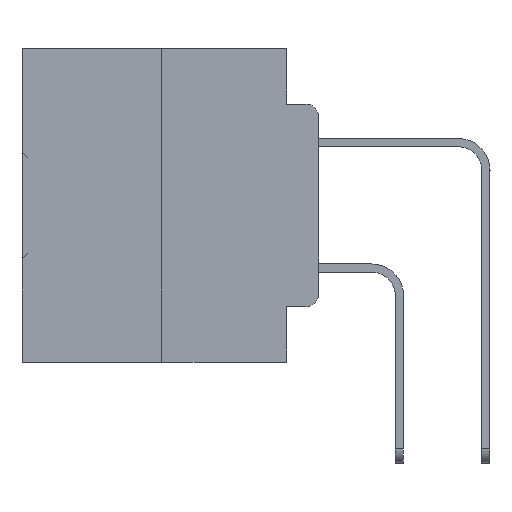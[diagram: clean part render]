
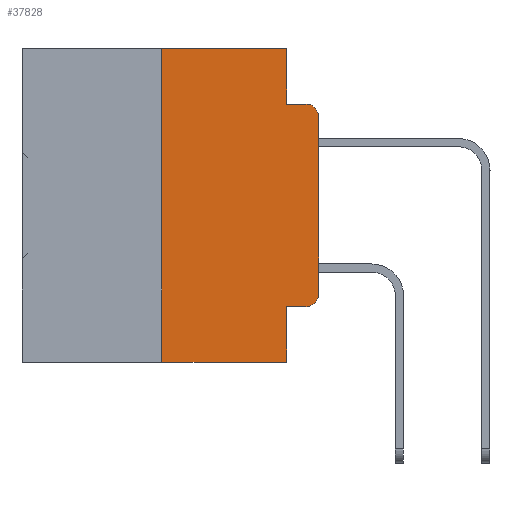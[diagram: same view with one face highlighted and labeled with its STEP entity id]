
A CAD part, left-side view. The second image highlights one B-rep face of the part: STEP entity #37828.
In plain terms, the highlighted planar face has unit normal (-1, 0, 0).
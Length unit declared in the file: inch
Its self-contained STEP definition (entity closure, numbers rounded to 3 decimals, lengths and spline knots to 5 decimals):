
#134 = DIRECTION ( 'NONE',  ( 0., 0., -1. ) ) ;
#221 = AXIS2_PLACEMENT_3D ( 'NONE', #33354, #1576, #6653 ) ;
#1245 = CARTESIAN_POINT ( 'NONE',  ( 0., 0., 0. ) ) ;
#1454 = LINE ( 'NONE', #13320, #4635 ) ;
#1519 = VERTEX_POINT ( 'NONE', #12803 ) ;
#1576 = DIRECTION ( 'NONE',  ( 1., 0., 0. ) ) ;
#2118 = CARTESIAN_POINT ( 'NONE',  ( 0., 0.473, 0. ) ) ;
#3173 = VECTOR ( 'NONE', #10102, 39.37008 ) ;
#4090 = CARTESIAN_POINT ( 'NONE',  ( 0., 0.051, 0. ) ) ;
#4349 = DIRECTION ( 'NONE',  ( 0., 0., 1. ) ) ;
#4635 = VECTOR ( 'NONE', #25233, 39.37008 ) ;
#6163 = EDGE_CURVE ( 'NONE', #16615, #1519, #25114, .T. ) ;
#6653 = DIRECTION ( 'NONE',  ( 0., 0., -1. ) ) ;
#6839 = VERTEX_POINT ( 'NONE', #30055 ) ;
#7775 = VECTOR ( 'NONE', #13465, 39.37008 ) ;
#8841 = CARTESIAN_POINT ( 'NONE',  ( 0., 0., -0.3915 ) ) ;
#9501 = DIRECTION ( 'NONE',  ( 0., 0., -1. ) ) ;
#9971 = AXIS2_PLACEMENT_3D ( 'NONE', #16643, #13518, #28905 ) ;
#10102 = DIRECTION ( 'NONE',  ( 0., 0., 1. ) ) ;
#11170 = VECTOR ( 'NONE', #9501, 39.37008 ) ;
#11258 = ORIENTED_EDGE ( 'NONE', *, *, #25419, .T. ) ;
#11680 = EDGE_CURVE ( 'NONE', #16615, #21361, #1454, .T. ) ;
#11742 = VECTOR ( 'NONE', #28440, 39.37008 ) ;
#12127 = ORIENTED_EDGE ( 'NONE', *, *, #31651, .T. ) ;
#12205 = CARTESIAN_POINT ( 'NONE',  ( 0., 0.051, 0. ) ) ;
#12661 = DIRECTION ( 'NONE',  ( 0., 0., -1. ) ) ;
#12803 = CARTESIAN_POINT ( 'NONE',  ( 0., 0.25, 0. ) ) ;
#12878 = ORIENTED_EDGE ( 'NONE', *, *, #6163, .F. ) ;
#13035 = VERTEX_POINT ( 'NONE', #8841 ) ;
#13320 = CARTESIAN_POINT ( 'NONE',  ( 0., 0.473, -0.5 ) ) ;
#13465 = DIRECTION ( 'NONE',  ( 0., -1., 0. ) ) ;
#13518 = DIRECTION ( 'NONE',  ( -1., 0., 0. ) ) ;
#15500 = CARTESIAN_POINT ( 'NONE',  ( 0., 0.051, -0.5 ) ) ;
#16203 = LINE ( 'NONE', #28486, #7775 ) ;
#16615 = VERTEX_POINT ( 'NONE', #28828 ) ;
#16643 = CARTESIAN_POINT ( 'NONE',  ( 0., 0.02, -0.3915 ) ) ;
#17129 = VECTOR ( 'NONE', #37710, 39.37008 ) ;
#18005 = EDGE_CURVE ( 'NONE', #13035, #23581, #22467, .T. ) ;
#18072 = LINE ( 'NONE', #12205, #11170 ) ;
#18110 = VECTOR ( 'NONE', #12661, 39.37008 ) ;
#18202 = CARTESIAN_POINT ( 'NONE',  ( 0., 0.051, -0.0885 ) ) ;
#18560 = CARTESIAN_POINT ( 'NONE',  ( 0., 0., -0.1085 ) ) ;
#18824 = EDGE_CURVE ( 'NONE', #28786, #34872, #37515, .T. ) ;
#18927 = FACE_OUTER_BOUND ( 'NONE', #23392, .T. ) ;
#19392 = CARTESIAN_POINT ( 'NONE',  ( 0., 0.051, 0. ) ) ;
#20721 = ORIENTED_EDGE ( 'NONE', *, *, #24501, .F. ) ;
#21201 = ORIENTED_EDGE ( 'NONE', *, *, #18824, .F. ) ;
#21361 = VERTEX_POINT ( 'NONE', #15500 ) ;
#21834 = LINE ( 'NONE', #4090, #18110 ) ;
#22467 = LINE ( 'NONE', #1245, #35851 ) ;
#22488 = ORIENTED_EDGE ( 'NONE', *, *, #37163, .F. ) ;
#22920 = CARTESIAN_POINT ( 'NONE',  ( 0., 0.02, -0.0885 ) ) ;
#23133 = AXIS2_PLACEMENT_3D ( 'NONE', #26811, #33236, #134 ) ;
#23392 = EDGE_LOOP ( 'NONE', ( #29933, #35490, #21201, #20721, #22488, #12878, #29882, #27152, #12127, #11258 ) ) ;
#23581 = VERTEX_POINT ( 'NONE', #18560 ) ;
#24501 = EDGE_CURVE ( 'NONE', #36699, #28786, #18072, .T. ) ;
#25114 = LINE ( 'NONE', #28042, #3173 ) ;
#25233 = DIRECTION ( 'NONE',  ( 0., -1., 0. ) ) ;
#25419 = EDGE_CURVE ( 'NONE', #26863, #13035, #26769, .T. ) ;
#26769 = CIRCLE ( 'NONE', #9971, 0.02 ) ;
#26811 = CARTESIAN_POINT ( 'NONE',  ( 0., 0.02, -0.1085 ) ) ;
#26863 = VERTEX_POINT ( 'NONE', #31688 ) ;
#27152 = ORIENTED_EDGE ( 'NONE', *, *, #27481, .F. ) ;
#27481 = EDGE_CURVE ( 'NONE', #6839, #21361, #21834, .T. ) ;
#28042 = CARTESIAN_POINT ( 'NONE',  ( 0., 0.25, 0. ) ) ;
#28385 = EDGE_CURVE ( 'NONE', #23581, #34872, #34352, .T. ) ;
#28440 = DIRECTION ( 'NONE',  ( 0., -1., 0. ) ) ;
#28486 = CARTESIAN_POINT ( 'NONE',  ( 0., 0.051, -0.4115 ) ) ;
#28786 = VERTEX_POINT ( 'NONE', #18202 ) ;
#28828 = CARTESIAN_POINT ( 'NONE',  ( 0., 0.25, -0.5 ) ) ;
#28905 = DIRECTION ( 'NONE',  ( 0., 0., -1. ) ) ;
#29882 = ORIENTED_EDGE ( 'NONE', *, *, #11680, .T. ) ;
#29933 = ORIENTED_EDGE ( 'NONE', *, *, #18005, .T. ) ;
#30055 = CARTESIAN_POINT ( 'NONE',  ( 0., 0.051, -0.4115 ) ) ;
#31651 = EDGE_CURVE ( 'NONE', #6839, #26863, #16203, .T. ) ;
#31688 = CARTESIAN_POINT ( 'NONE',  ( 0., 0.02, -0.4115 ) ) ;
#33236 = DIRECTION ( 'NONE',  ( -1., 0., 0. ) ) ;
#33354 = CARTESIAN_POINT ( 'NONE',  ( 0., 0.473, 0. ) ) ;
#33542 = PLANE ( 'NONE',  #221 ) ;
#34352 = CIRCLE ( 'NONE', #23133, 0.02 ) ;
#34598 = CARTESIAN_POINT ( 'NONE',  ( 0., 0.051, -0.0885 ) ) ;
#34872 = VERTEX_POINT ( 'NONE', #22920 ) ;
#35049 = LINE ( 'NONE', #2118, #11742 ) ;
#35490 = ORIENTED_EDGE ( 'NONE', *, *, #28385, .T. ) ;
#35851 = VECTOR ( 'NONE', #4349, 39.37008 ) ;
#36699 = VERTEX_POINT ( 'NONE', #19392 ) ;
#37163 = EDGE_CURVE ( 'NONE', #1519, #36699, #35049, .T. ) ;
#37515 = LINE ( 'NONE', #34598, #17129 ) ;
#37710 = DIRECTION ( 'NONE',  ( 0., -1., 0. ) ) ;
#37828 = ADVANCED_FACE ( 'NONE', ( #18927 ), #33542, .F. ) ;
